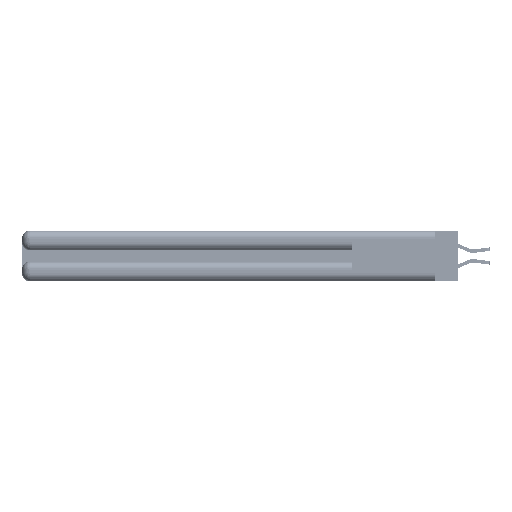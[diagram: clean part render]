
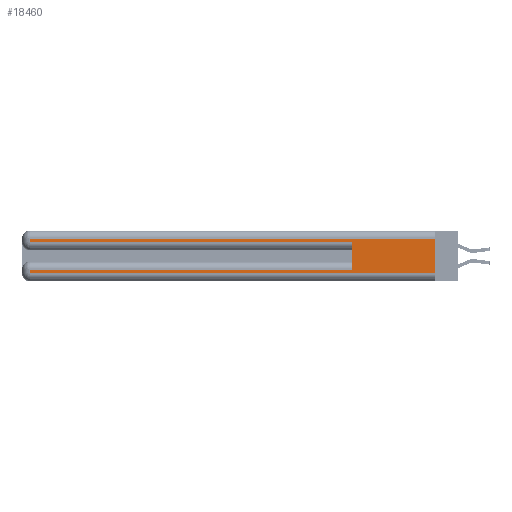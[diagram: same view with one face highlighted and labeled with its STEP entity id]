
A CAD part, left-side view. The second image highlights one B-rep face of the part: STEP entity #18460.
In plain terms, the highlighted planar face has unit normal (-1, 0, 0).
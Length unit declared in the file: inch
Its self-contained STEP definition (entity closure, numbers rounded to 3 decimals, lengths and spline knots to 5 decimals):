
#636 = ORIENTED_EDGE ( 'NONE', *, *, #21735, .F. ) ;
#1407 = CARTESIAN_POINT ( 'NONE',  ( 0., 0., 0.37 ) ) ;
#2997 = EDGE_CURVE ( 'NONE', #7043, #33329, #38019, .T. ) ;
#3509 = VERTEX_POINT ( 'NONE', #5942 ) ;
#4155 = ORIENTED_EDGE ( 'NONE', *, *, #14121, .T. ) ;
#4213 = ORIENTED_EDGE ( 'NONE', *, *, #40200, .T. ) ;
#4665 = DIRECTION ( 'NONE',  ( 1., 0., 0. ) ) ;
#4738 = DIRECTION ( 'NONE',  ( 0., 0., -1. ) ) ;
#5942 = CARTESIAN_POINT ( 'NONE',  ( 0., 0., 0.31 ) ) ;
#7043 = VERTEX_POINT ( 'NONE', #9659 ) ;
#9222 = EDGE_CURVE ( 'NONE', #3509, #22085, #19204, .T. ) ;
#9659 = CARTESIAN_POINT ( 'NONE',  ( 0., 2.94, 0.085 ) ) ;
#9959 = DIRECTION ( 'NONE',  ( 0., 1., 0. ) ) ;
#10594 = EDGE_LOOP ( 'NONE', ( #33282, #37749, #42080, #4155, #636, #31139, #15175, #4213 ) ) ;
#12483 = LINE ( 'NONE', #30248, #19107 ) ;
#12827 = EDGE_CURVE ( 'NONE', #14648, #35223, #40337, .T. ) ;
#13416 = AXIS2_PLACEMENT_3D ( 'NONE', #1407, #4665, #33057 ) ;
#14121 = EDGE_CURVE ( 'NONE', #35223, #34328, #21368, .T. ) ;
#14648 = VERTEX_POINT ( 'NONE', #22209 ) ;
#14747 = VECTOR ( 'NONE', #4738, 39.37008 ) ;
#15175 = ORIENTED_EDGE ( 'NONE', *, *, #2997, .T. ) ;
#15862 = LINE ( 'NONE', #37803, #45722 ) ;
#16889 = CARTESIAN_POINT ( 'NONE',  ( 0., 2.94, 0.06 ) ) ;
#17074 = DIRECTION ( 'NONE',  ( 0., 0., -1. ) ) ;
#17220 = CARTESIAN_POINT ( 'NONE',  ( 0., 2.94, 0.37 ) ) ;
#17288 = DIRECTION ( 'NONE',  ( 0., 0., 1. ) ) ;
#17597 = VECTOR ( 'NONE', #17288, 39.37008 ) ;
#17991 = CARTESIAN_POINT ( 'NONE',  ( 0., 0., 0.06 ) ) ;
#18460 = ADVANCED_FACE ( 'NONE', ( #22031 ), #33223, .F. ) ;
#19107 = VECTOR ( 'NONE', #22270, 39.37008 ) ;
#19204 = LINE ( 'NONE', #34977, #34688 ) ;
#19923 = CARTESIAN_POINT ( 'NONE',  ( 0., 0.6, 0.145 ) ) ;
#21368 = LINE ( 'NONE', #35895, #29110 ) ;
#21521 = DIRECTION ( 'NONE',  ( 0., -1., 0. ) ) ;
#21735 = EDGE_CURVE ( 'NONE', #28291, #34328, #25288, .T. ) ;
#22031 = FACE_OUTER_BOUND ( 'NONE', #10594, .T. ) ;
#22085 = VERTEX_POINT ( 'NONE', #17991 ) ;
#22209 = CARTESIAN_POINT ( 'NONE',  ( 0., 2.94, 0.31 ) ) ;
#22270 = DIRECTION ( 'NONE',  ( 0., 1., 0. ) ) ;
#22912 = EDGE_CURVE ( 'NONE', #28291, #7043, #15862, .T. ) ;
#23174 = EDGE_CURVE ( 'NONE', #3509, #14648, #12483, .T. ) ;
#25288 = LINE ( 'NONE', #19923, #17597 ) ;
#25506 = CARTESIAN_POINT ( 'NONE',  ( 0., 0.6, 0.285 ) ) ;
#26178 = CARTESIAN_POINT ( 'NONE',  ( 0., 2.94, 0.37 ) ) ;
#27446 = CARTESIAN_POINT ( 'NONE',  ( 0., 2.94, 0.285 ) ) ;
#28291 = VERTEX_POINT ( 'NONE', #32502 ) ;
#29110 = VECTOR ( 'NONE', #21521, 39.37008 ) ;
#29861 = VECTOR ( 'NONE', #43322, 39.37008 ) ;
#29979 = DIRECTION ( 'NONE',  ( 0., -1., 0. ) ) ;
#30248 = CARTESIAN_POINT ( 'NONE',  ( 0., 0., 0.31 ) ) ;
#31139 = ORIENTED_EDGE ( 'NONE', *, *, #22912, .T. ) ;
#32502 = CARTESIAN_POINT ( 'NONE',  ( 0., 0.6, 0.085 ) ) ;
#33057 = DIRECTION ( 'NONE',  ( 0., 0., -1. ) ) ;
#33223 = PLANE ( 'NONE',  #13416 ) ;
#33282 = ORIENTED_EDGE ( 'NONE', *, *, #9222, .F. ) ;
#33329 = VERTEX_POINT ( 'NONE', #16889 ) ;
#34000 = VECTOR ( 'NONE', #29979, 39.37008 ) ;
#34328 = VERTEX_POINT ( 'NONE', #25506 ) ;
#34688 = VECTOR ( 'NONE', #17074, 39.37008 ) ;
#34977 = CARTESIAN_POINT ( 'NONE',  ( 0., 0., 0.37 ) ) ;
#35223 = VERTEX_POINT ( 'NONE', #27446 ) ;
#35895 = CARTESIAN_POINT ( 'NONE',  ( 0., 0., 0.285 ) ) ;
#37041 = CARTESIAN_POINT ( 'NONE',  ( 0., 0., 0.06 ) ) ;
#37749 = ORIENTED_EDGE ( 'NONE', *, *, #23174, .T. ) ;
#37803 = CARTESIAN_POINT ( 'NONE',  ( 0., 0., 0.085 ) ) ;
#38019 = LINE ( 'NONE', #26178, #14747 ) ;
#40200 = EDGE_CURVE ( 'NONE', #33329, #22085, #43382, .T. ) ;
#40337 = LINE ( 'NONE', #17220, #29861 ) ;
#42080 = ORIENTED_EDGE ( 'NONE', *, *, #12827, .T. ) ;
#43322 = DIRECTION ( 'NONE',  ( 0., 0., -1. ) ) ;
#43382 = LINE ( 'NONE', #37041, #34000 ) ;
#45722 = VECTOR ( 'NONE', #9959, 39.37008 ) ;
